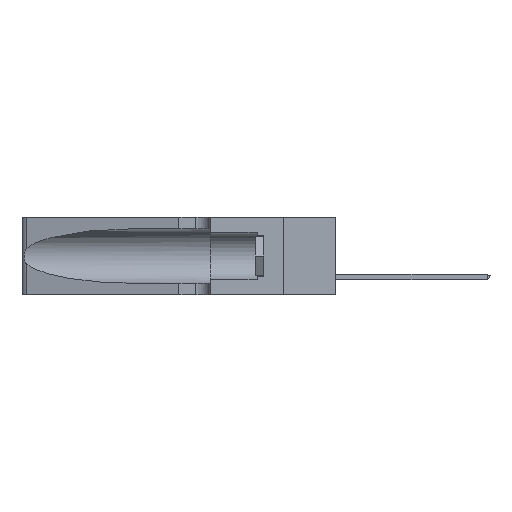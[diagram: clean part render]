
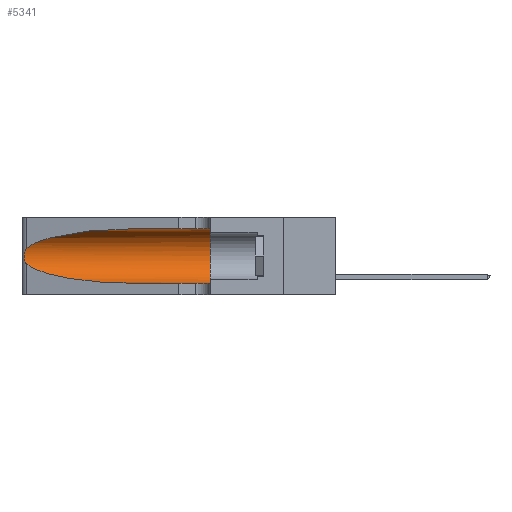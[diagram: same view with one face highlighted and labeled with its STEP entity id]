
A CAD part, left-side view. The second image highlights one B-rep face of the part: STEP entity #5341.
In plain terms, the highlighted cylindrical face has radius 3.308 mm (diameter 6.617 mm), a partial arc.
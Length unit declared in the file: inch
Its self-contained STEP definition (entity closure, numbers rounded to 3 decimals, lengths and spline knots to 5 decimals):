
#826 = DIRECTION ( 'NONE',  ( 0., -1., 0. ) ) ;
#999 = CARTESIAN_POINT ( 'NONE',  ( 0.26075, 1.23896, 0.19203 ) ) ;
#1273 = CARTESIAN_POINT ( 'NONE',  ( 0.1305, 0.72297, 0.05475 ) ) ;
#2555 = CARTESIAN_POINT ( 'NONE',  ( 0.25487, 1.22718, 0.22369 ) ) ;
#2877 = ORIENTED_EDGE ( 'NONE', *, *, #22743, .T. ) ;
#3086 = CARTESIAN_POINT ( 'NONE',  ( 0.25487, 1.22718, 0.22369 ) ) ;
#3197 = CARTESIAN_POINT ( 'NONE',  ( 0.26075, 1.23896, 0.178 ) ) ;
#3510 = CARTESIAN_POINT ( 'NONE',  ( 0.25639, 1.23184, 0.21858 ) ) ;
#3714 = EDGE_CURVE ( 'NONE', #8034, #12327, #22050, .T. ) ;
#5169 = VERTEX_POINT ( 'NONE', #11417 ) ;
#5208 = B_SPLINE_CURVE_WITH_KNOTS ( 'NONE', 3,
 ( #3086, #8069, #3510, #13030, #10805, #30186, #999, #3197, #10584, #29854, #25288, #20209, #22970, #8487 ),
 .UNSPECIFIED., .F., .F.,
 ( 4, 2, 2, 2, 2, 2, 4 ),
 ( 0., 0.00027, 0.00053, 0.00107, 0.0016, 0.00187, 0.00214 ),
 .UNSPECIFIED. ) ;
#5341 = ADVANCED_FACE ( 'NONE', ( #21944 ), #15126, .F. ) ;
#5379 = DIRECTION ( 'NONE',  ( 0., 1., 0. ) ) ;
#6827 = ORIENTED_EDGE ( 'NONE', *, *, #9342, .F. ) ;
#7377 = CARTESIAN_POINT ( 'NONE',  ( 0.2373, 1.15595, 0.08982 ) ) ;
#7486 = LINE ( 'NONE', #12864, #8617 ) ;
#7551 =( BOUNDED_CURVE ( )  B_SPLINE_CURVE ( 3, ( #14983, #24422, #29410, #2555 ),
 .UNSPECIFIED., .F., .F. ) 
 B_SPLINE_CURVE_WITH_KNOTS ( ( 4, 4 ),
 ( 1.5708, 2.84003 ),
 .UNSPECIFIED. ) 
 CURVE ( )  GEOMETRIC_REPRESENTATION_ITEM ( )  RATIONAL_B_SPLINE_CURVE ( ( 1., 0.87, 0.87, 1. ) ) 
 REPRESENTATION_ITEM ( '' )  );
#8034 = VERTEX_POINT ( 'NONE', #1273 ) ;
#8069 = CARTESIAN_POINT ( 'NONE',  ( 0.25555, 1.22994, 0.2215 ) ) ;
#8487 = CARTESIAN_POINT ( 'NONE',  ( 0.25487, 1.22718, 0.14631 ) ) ;
#8617 = VECTOR ( 'NONE', #826, 39.37008 ) ;
#9185 = CARTESIAN_POINT ( 'NONE',  ( 0.25487, 1.22718, 0.14631 ) ) ;
#9342 = EDGE_CURVE ( 'NONE', #17959, #12327, #14265, .T. ) ;
#9469 = DIRECTION ( 'NONE',  ( 0., -1., 0. ) ) ;
#10553 = ORIENTED_EDGE ( 'NONE', *, *, #15990, .F. ) ;
#10584 = CARTESIAN_POINT ( 'NONE',  ( 0.26017, 1.23833, 0.17102 ) ) ;
#10805 = CARTESIAN_POINT ( 'NONE',  ( 0.25854, 1.2359, 0.20912 ) ) ;
#11270 = DIRECTION ( 'NONE',  ( 0., -1., 0. ) ) ;
#11417 = CARTESIAN_POINT ( 'NONE',  ( 0.25487, 1.22718, 0.14631 ) ) ;
#11496 = CARTESIAN_POINT ( 'NONE',  ( 0.1305, 1.61858, 0.185 ) ) ;
#11631 = CARTESIAN_POINT ( 'NONE',  ( 0.18966, 0.96281, 0.05475 ) ) ;
#11996 = ORIENTED_EDGE ( 'NONE', *, *, #30038, .T. ) ;
#12327 = VERTEX_POINT ( 'NONE', #13063 ) ;
#12864 = CARTESIAN_POINT ( 'NONE',  ( 0.1305, 1.61858, 0.31525 ) ) ;
#13030 = CARTESIAN_POINT ( 'NONE',  ( 0.25787, 1.23484, 0.2124 ) ) ;
#13063 = CARTESIAN_POINT ( 'NONE',  ( 0.1305, 0.35, 0.05475 ) ) ;
#13380 = CARTESIAN_POINT ( 'NONE',  ( 0.25487, 1.22718, 0.22369 ) ) ;
#14265 = CIRCLE ( 'NONE', #14411, 0.13025 ) ;
#14411 = AXIS2_PLACEMENT_3D ( 'NONE', #14988, #5379, #19855 ) ;
#14983 = CARTESIAN_POINT ( 'NONE',  ( 0.1305, 0.72297, 0.31525 ) ) ;
#14988 = CARTESIAN_POINT ( 'NONE',  ( 0.1305, 0.35, 0.185 ) ) ;
#15126 = CYLINDRICAL_SURFACE ( 'NONE', #23629, 0.13025 ) ;
#15990 = EDGE_CURVE ( 'NONE', #18329, #17959, #7486, .T. ) ;
#16854 = ORIENTED_EDGE ( 'NONE', *, *, #24905, .T. ) ;
#17152 = VECTOR ( 'NONE', #9469, 39.37008 ) ;
#17959 = VERTEX_POINT ( 'NONE', #20787 ) ;
#18329 = VERTEX_POINT ( 'NONE', #30658 ) ;
#18383 = ORIENTED_EDGE ( 'NONE', *, *, #3714, .T. ) ;
#18831 =( BOUNDED_CURVE ( )  B_SPLINE_CURVE ( 3, ( #9185, #7377, #11631, #26083 ),
 .UNSPECIFIED., .F., .F. ) 
 B_SPLINE_CURVE_WITH_KNOTS ( ( 4, 4 ),
 ( 3.44316, 4.71239 ),
 .UNSPECIFIED. ) 
 CURVE ( )  GEOMETRIC_REPRESENTATION_ITEM ( )  RATIONAL_B_SPLINE_CURVE ( ( 1., 0.87, 0.87, 1. ) ) 
 REPRESENTATION_ITEM ( '' )  );
#19855 = DIRECTION ( 'NONE',  ( 0., 0., 1. ) ) ;
#20209 = CARTESIAN_POINT ( 'NONE',  ( 0.25639, 1.23186, 0.15144 ) ) ;
#20787 = CARTESIAN_POINT ( 'NONE',  ( 0.1305, 0.35, 0.31525 ) ) ;
#21944 = FACE_OUTER_BOUND ( 'NONE', #26391, .T. ) ;
#22050 = LINE ( 'NONE', #28936, #17152 ) ;
#22743 = EDGE_CURVE ( 'NONE', #18329, #31262, #7551, .T. ) ;
#22970 = CARTESIAN_POINT ( 'NONE',  ( 0.25555, 1.22993, 0.14849 ) ) ;
#23629 = AXIS2_PLACEMENT_3D ( 'NONE', #11496, #11270, #28424 ) ;
#24422 = CARTESIAN_POINT ( 'NONE',  ( 0.18966, 0.96281, 0.31525 ) ) ;
#24905 = EDGE_CURVE ( 'NONE', #5169, #8034, #18831, .T. ) ;
#25288 = CARTESIAN_POINT ( 'NONE',  ( 0.25789, 1.23486, 0.15765 ) ) ;
#26083 = CARTESIAN_POINT ( 'NONE',  ( 0.1305, 0.72297, 0.05475 ) ) ;
#26391 = EDGE_LOOP ( 'NONE', ( #2877, #11996, #16854, #18383, #6827, #10553 ) ) ;
#28424 = DIRECTION ( 'NONE',  ( 0., 0., -1. ) ) ;
#28936 = CARTESIAN_POINT ( 'NONE',  ( 0.1305, 1.61858, 0.05475 ) ) ;
#29410 = CARTESIAN_POINT ( 'NONE',  ( 0.2373, 1.15595, 0.28018 ) ) ;
#29854 = CARTESIAN_POINT ( 'NONE',  ( 0.25856, 1.23593, 0.16098 ) ) ;
#30038 = EDGE_CURVE ( 'NONE', #31262, #5169, #5208, .T. ) ;
#30186 = CARTESIAN_POINT ( 'NONE',  ( 0.26018, 1.23835, 0.19895 ) ) ;
#30658 = CARTESIAN_POINT ( 'NONE',  ( 0.1305, 0.72297, 0.31525 ) ) ;
#31262 = VERTEX_POINT ( 'NONE', #13380 ) ;
